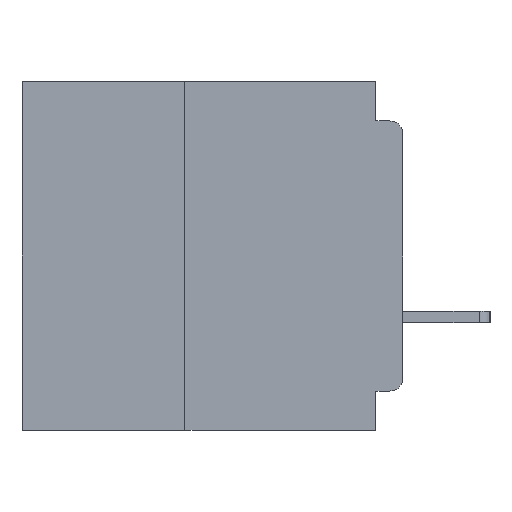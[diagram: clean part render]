
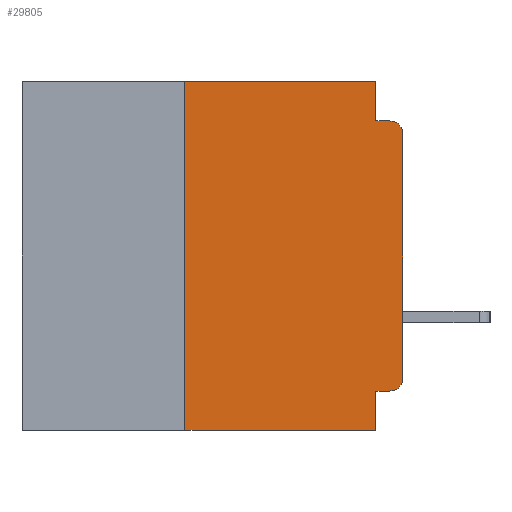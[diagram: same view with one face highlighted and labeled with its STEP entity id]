
A CAD part, left-side view. The second image highlights one B-rep face of the part: STEP entity #29805.
In plain terms, the highlighted planar face has unit normal (-1, 0, 0).
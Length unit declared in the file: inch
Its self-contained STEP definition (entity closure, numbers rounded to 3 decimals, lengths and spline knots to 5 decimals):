
#380 = AXIS2_PLACEMENT_3D ( 'NONE', #33546, #13194, #36982 ) ;
#643 = VECTOR ( 'NONE', #16532, 39.37008 ) ;
#1918 = CARTESIAN_POINT ( 'NONE',  ( 0., 0.031, -0.4 ) ) ;
#1978 = DIRECTION ( 'NONE',  ( -1., 0., 0. ) ) ;
#2660 = DIRECTION ( 'NONE',  ( 0., 0., -1. ) ) ;
#3171 = DIRECTION ( 'NONE',  ( 0., -1., 0. ) ) ;
#3298 = ORIENTED_EDGE ( 'NONE', *, *, #13366, .F. ) ;
#4614 = EDGE_LOOP ( 'NONE', ( #34967, #38716, #27451, #3298, #39971, #8179, #19335, #33377, #14207, #32143 ) ) ;
#5732 = VERTEX_POINT ( 'NONE', #8620 ) ;
#6008 = CARTESIAN_POINT ( 'NONE',  ( 0., 0.437, -0.4 ) ) ;
#6063 = CIRCLE ( 'NONE', #6470, 0.015 ) ;
#6470 = AXIS2_PLACEMENT_3D ( 'NONE', #22541, #1978, #25960 ) ;
#8179 = ORIENTED_EDGE ( 'NONE', *, *, #11055, .F. ) ;
#8620 = CARTESIAN_POINT ( 'NONE',  ( 0., 0., -0.34 ) ) ;
#8692 = EDGE_CURVE ( 'NONE', #32055, #25738, #24042, .T. ) ;
#9401 = VECTOR ( 'NONE', #31475, 39.37008 ) ;
#11055 = EDGE_CURVE ( 'NONE', #32055, #14046, #28582, .T. ) ;
#11088 = VERTEX_POINT ( 'NONE', #31783 ) ;
#11301 = CARTESIAN_POINT ( 'NONE',  ( 0., 0., -0.06 ) ) ;
#11395 = CARTESIAN_POINT ( 'NONE',  ( 0., 0.015, -0.355 ) ) ;
#11446 = DIRECTION ( 'NONE',  ( 0., -1., 0. ) ) ;
#11640 = VERTEX_POINT ( 'NONE', #11395 ) ;
#13194 = DIRECTION ( 'NONE',  ( -1., 0., 0. ) ) ;
#13366 = EDGE_CURVE ( 'NONE', #13858, #11088, #25862, .T. ) ;
#13388 = CARTESIAN_POINT ( 'NONE',  ( 0., 0.25, 0. ) ) ;
#13858 = VERTEX_POINT ( 'NONE', #22552 ) ;
#14046 = VERTEX_POINT ( 'NONE', #13388 ) ;
#14207 = ORIENTED_EDGE ( 'NONE', *, *, #44142, .F. ) ;
#14528 = VERTEX_POINT ( 'NONE', #26201 ) ;
#14558 = CARTESIAN_POINT ( 'NONE',  ( 0., 0.25, -0.4 ) ) ;
#14932 = VECTOR ( 'NONE', #2660, 39.37008 ) ;
#15019 = DIRECTION ( 'NONE',  ( 0., 0., 1. ) ) ;
#15027 = VECTOR ( 'NONE', #19785, 39.37008 ) ;
#15352 = LINE ( 'NONE', #21507, #31271 ) ;
#15572 = VERTEX_POINT ( 'NONE', #11301 ) ;
#16446 = VECTOR ( 'NONE', #3171, 39.37008 ) ;
#16532 = DIRECTION ( 'NONE',  ( 0., 0., -1. ) ) ;
#16639 = DIRECTION ( 'NONE',  ( 1., 0., 0. ) ) ;
#18207 = EDGE_CURVE ( 'NONE', #11088, #14528, #25462, .T. ) ;
#19037 = CIRCLE ( 'NONE', #380, 0.015 ) ;
#19335 = ORIENTED_EDGE ( 'NONE', *, *, #8692, .T. ) ;
#19785 = DIRECTION ( 'NONE',  ( 0., -1., 0. ) ) ;
#19789 = CARTESIAN_POINT ( 'NONE',  ( 0., 0.031, -0.4 ) ) ;
#20454 = VERTEX_POINT ( 'NONE', #35156 ) ;
#21310 = EDGE_CURVE ( 'NONE', #11640, #5732, #6063, .T. ) ;
#21507 = CARTESIAN_POINT ( 'NONE',  ( 0., 0.437, 0. ) ) ;
#21623 = CARTESIAN_POINT ( 'NONE',  ( 0., 0., -0.355 ) ) ;
#22541 = CARTESIAN_POINT ( 'NONE',  ( 0., 0.015, -0.34 ) ) ;
#22552 = CARTESIAN_POINT ( 'NONE',  ( 0., 0.031, 0. ) ) ;
#22773 = VECTOR ( 'NONE', #15019, 39.37008 ) ;
#23677 = CARTESIAN_POINT ( 'NONE',  ( 0., 0., -0.045 ) ) ;
#24042 = LINE ( 'NONE', #6008, #15027 ) ;
#24964 = EDGE_CURVE ( 'NONE', #14046, #13858, #15352, .T. ) ;
#25462 = LINE ( 'NONE', #23677, #16446 ) ;
#25738 = VERTEX_POINT ( 'NONE', #1918 ) ;
#25862 = LINE ( 'NONE', #33503, #643 ) ;
#25960 = DIRECTION ( 'NONE',  ( 0., 0., -1. ) ) ;
#26201 = CARTESIAN_POINT ( 'NONE',  ( 0., 0.015, -0.045 ) ) ;
#26695 = CARTESIAN_POINT ( 'NONE',  ( 0., 0.437, 0. ) ) ;
#27451 = ORIENTED_EDGE ( 'NONE', *, *, #18207, .F. ) ;
#28582 = LINE ( 'NONE', #14558, #9401 ) ;
#29805 = ADVANCED_FACE ( 'NONE', ( #43122 ), #37047, .F. ) ;
#31271 = VECTOR ( 'NONE', #11446, 39.37008 ) ;
#31475 = DIRECTION ( 'NONE',  ( 0., 0., 1. ) ) ;
#31783 = CARTESIAN_POINT ( 'NONE',  ( 0., 0.031, -0.045 ) ) ;
#31847 = LINE ( 'NONE', #38819, #22773 ) ;
#32055 = VERTEX_POINT ( 'NONE', #33147 ) ;
#32143 = ORIENTED_EDGE ( 'NONE', *, *, #21310, .T. ) ;
#32738 = EDGE_CURVE ( 'NONE', #15572, #14528, #19037, .T. ) ;
#33147 = CARTESIAN_POINT ( 'NONE',  ( 0., 0.25, -0.4 ) ) ;
#33377 = ORIENTED_EDGE ( 'NONE', *, *, #41560, .F. ) ;
#33503 = CARTESIAN_POINT ( 'NONE',  ( 0., 0.031, 0. ) ) ;
#33546 = CARTESIAN_POINT ( 'NONE',  ( 0., 0.015, -0.06 ) ) ;
#34449 = VECTOR ( 'NONE', #35207, 39.37008 ) ;
#34967 = ORIENTED_EDGE ( 'NONE', *, *, #36480, .T. ) ;
#35156 = CARTESIAN_POINT ( 'NONE',  ( 0., 0.031, -0.355 ) ) ;
#35207 = DIRECTION ( 'NONE',  ( 0., 1., 0. ) ) ;
#35498 = LINE ( 'NONE', #21623, #34449 ) ;
#36480 = EDGE_CURVE ( 'NONE', #5732, #15572, #31847, .T. ) ;
#36982 = DIRECTION ( 'NONE',  ( 0., 0., -1. ) ) ;
#37047 = PLANE ( 'NONE',  #41910 ) ;
#38716 = ORIENTED_EDGE ( 'NONE', *, *, #32738, .T. ) ;
#38819 = CARTESIAN_POINT ( 'NONE',  ( 0., 0., 0. ) ) ;
#39971 = ORIENTED_EDGE ( 'NONE', *, *, #24964, .F. ) ;
#40460 = DIRECTION ( 'NONE',  ( 0., 0., -1. ) ) ;
#41560 = EDGE_CURVE ( 'NONE', #20454, #25738, #42082, .T. ) ;
#41910 = AXIS2_PLACEMENT_3D ( 'NONE', #26695, #16639, #40460 ) ;
#42082 = LINE ( 'NONE', #19789, #14932 ) ;
#43122 = FACE_OUTER_BOUND ( 'NONE', #4614, .T. ) ;
#44142 = EDGE_CURVE ( 'NONE', #11640, #20454, #35498, .T. ) ;
